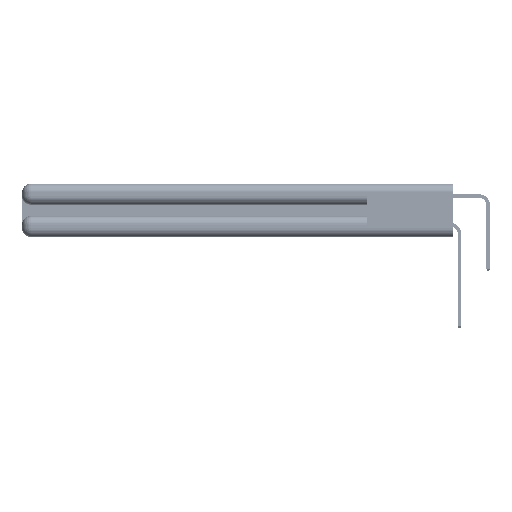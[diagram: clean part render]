
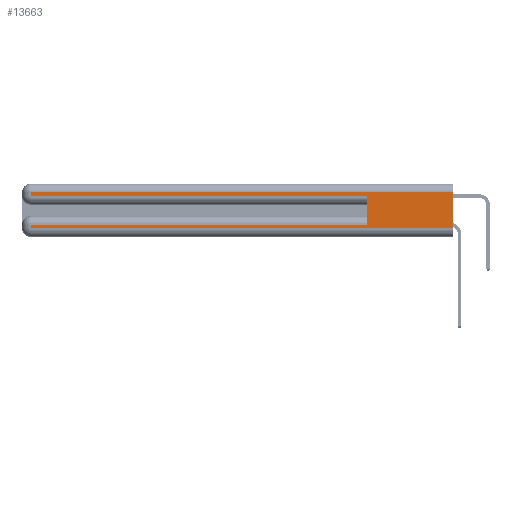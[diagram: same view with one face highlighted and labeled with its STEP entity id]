
A CAD part, left-side view. The second image highlights one B-rep face of the part: STEP entity #13663.
In plain terms, the highlighted planar face has unit normal (-1, 0, 0).
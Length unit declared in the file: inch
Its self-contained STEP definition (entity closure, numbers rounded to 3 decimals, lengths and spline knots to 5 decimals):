
#2022 = VECTOR ( 'NONE', #15701, 39.37008 ) ;
#2700 = VECTOR ( 'NONE', #13533, 39.37008 ) ;
#2870 = ORIENTED_EDGE ( 'NONE', *, *, #15975, .T. ) ;
#3063 = CARTESIAN_POINT ( 'NONE',  ( 0., 0., 0.37 ) ) ;
#3292 = CARTESIAN_POINT ( 'NONE',  ( 0., 2.94, 0.37 ) ) ;
#3573 = ORIENTED_EDGE ( 'NONE', *, *, #9016, .T. ) ;
#4282 = EDGE_CURVE ( 'NONE', #10312, #24554, #9571, .T. ) ;
#5834 = CARTESIAN_POINT ( 'NONE',  ( 0., 0., 0.31 ) ) ;
#7345 = ORIENTED_EDGE ( 'NONE', *, *, #32554, .T. ) ;
#7349 = VERTEX_POINT ( 'NONE', #16897 ) ;
#9016 = EDGE_CURVE ( 'NONE', #26921, #52158, #13881, .T. ) ;
#9571 = LINE ( 'NONE', #3292, #41590 ) ;
#10312 = VERTEX_POINT ( 'NONE', #43508 ) ;
#10549 = EDGE_CURVE ( 'NONE', #16069, #52158, #14467, .T. ) ;
#10776 = DIRECTION ( 'NONE',  ( 0., 0., -1. ) ) ;
#13320 = CARTESIAN_POINT ( 'NONE',  ( 0., 0., 0.285 ) ) ;
#13533 = DIRECTION ( 'NONE',  ( 0., 1., 0. ) ) ;
#13663 = ADVANCED_FACE ( 'NONE', ( #46387 ), #17397, .F. ) ;
#13881 = LINE ( 'NONE', #13320, #35405 ) ;
#13974 = ORIENTED_EDGE ( 'NONE', *, *, #4282, .T. ) ;
#14254 = DIRECTION ( 'NONE',  ( 1., 0., 0. ) ) ;
#14407 = CARTESIAN_POINT ( 'NONE',  ( 0., 2.94, 0.06 ) ) ;
#14467 = LINE ( 'NONE', #53503, #36682 ) ;
#15701 = DIRECTION ( 'NONE',  ( 0., 0., -1. ) ) ;
#15975 = EDGE_CURVE ( 'NONE', #7349, #54099, #26243, .T. ) ;
#16069 = VERTEX_POINT ( 'NONE', #51328 ) ;
#16101 = DIRECTION ( 'NONE',  ( 0., 0., 1. ) ) ;
#16160 = EDGE_CURVE ( 'NONE', #16069, #10312, #24245, .T. ) ;
#16296 = EDGE_CURVE ( 'NONE', #7349, #32744, #47093, .T. ) ;
#16897 = CARTESIAN_POINT ( 'NONE',  ( 0., 0., 0.31 ) ) ;
#17177 = CARTESIAN_POINT ( 'NONE',  ( 0., 2.94, 0.31 ) ) ;
#17397 = PLANE ( 'NONE',  #47474 ) ;
#18087 = VECTOR ( 'NONE', #35517, 39.37008 ) ;
#19049 = VECTOR ( 'NONE', #22633, 39.37008 ) ;
#21220 = CARTESIAN_POINT ( 'NONE',  ( 0., 0.6, 0.285 ) ) ;
#22367 = CARTESIAN_POINT ( 'NONE',  ( 0., 2.94, 0.37 ) ) ;
#22633 = DIRECTION ( 'NONE',  ( 0., 1., 0. ) ) ;
#23081 = EDGE_CURVE ( 'NONE', #54099, #26921, #23910, .T. ) ;
#23487 = VECTOR ( 'NONE', #26236, 39.37008 ) ;
#23910 = LINE ( 'NONE', #22367, #18087 ) ;
#24245 = LINE ( 'NONE', #43831, #19049 ) ;
#24554 = VERTEX_POINT ( 'NONE', #14407 ) ;
#26236 = DIRECTION ( 'NONE',  ( 0., -1., 0. ) ) ;
#26243 = LINE ( 'NONE', #5834, #2700 ) ;
#26921 = VERTEX_POINT ( 'NONE', #52106 ) ;
#32554 = EDGE_CURVE ( 'NONE', #24554, #32744, #33982, .T. ) ;
#32744 = VERTEX_POINT ( 'NONE', #52719 ) ;
#32913 = DIRECTION ( 'NONE',  ( 0., 0., -1. ) ) ;
#33920 = CARTESIAN_POINT ( 'NONE',  ( 0., 0., 0.06 ) ) ;
#33982 = LINE ( 'NONE', #33920, #23487 ) ;
#35405 = VECTOR ( 'NONE', #42716, 39.37008 ) ;
#35517 = DIRECTION ( 'NONE',  ( 0., 0., -1. ) ) ;
#36682 = VECTOR ( 'NONE', #16101, 39.37008 ) ;
#38362 = CARTESIAN_POINT ( 'NONE',  ( 0., 0., 0.37 ) ) ;
#41590 = VECTOR ( 'NONE', #32913, 39.37008 ) ;
#42716 = DIRECTION ( 'NONE',  ( 0., -1., 0. ) ) ;
#43508 = CARTESIAN_POINT ( 'NONE',  ( 0., 2.94, 0.085 ) ) ;
#43831 = CARTESIAN_POINT ( 'NONE',  ( 0., 0., 0.085 ) ) ;
#44235 = ORIENTED_EDGE ( 'NONE', *, *, #10549, .F. ) ;
#46387 = FACE_OUTER_BOUND ( 'NONE', #51863, .T. ) ;
#47093 = LINE ( 'NONE', #3063, #2022 ) ;
#47474 = AXIS2_PLACEMENT_3D ( 'NONE', #38362, #14254, #10776 ) ;
#47764 = ORIENTED_EDGE ( 'NONE', *, *, #23081, .T. ) ;
#51328 = CARTESIAN_POINT ( 'NONE',  ( 0., 0.6, 0.085 ) ) ;
#51863 = EDGE_LOOP ( 'NONE', ( #52403, #2870, #47764, #3573, #44235, #52274, #13974, #7345 ) ) ;
#52106 = CARTESIAN_POINT ( 'NONE',  ( 0., 2.94, 0.285 ) ) ;
#52158 = VERTEX_POINT ( 'NONE', #21220 ) ;
#52274 = ORIENTED_EDGE ( 'NONE', *, *, #16160, .T. ) ;
#52403 = ORIENTED_EDGE ( 'NONE', *, *, #16296, .F. ) ;
#52719 = CARTESIAN_POINT ( 'NONE',  ( 0., 0., 0.06 ) ) ;
#53503 = CARTESIAN_POINT ( 'NONE',  ( 0., 0.6, 0.145 ) ) ;
#54099 = VERTEX_POINT ( 'NONE', #17177 ) ;
